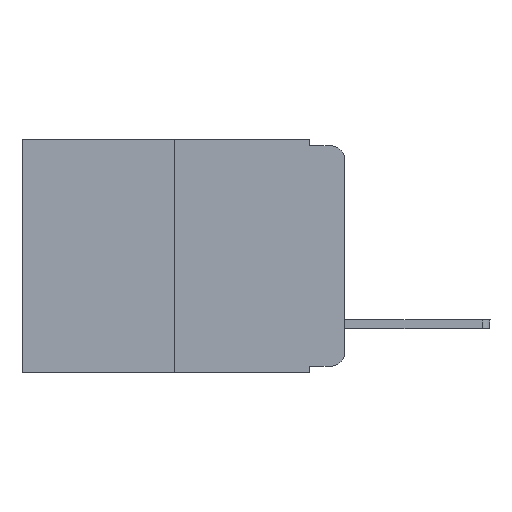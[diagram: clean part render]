
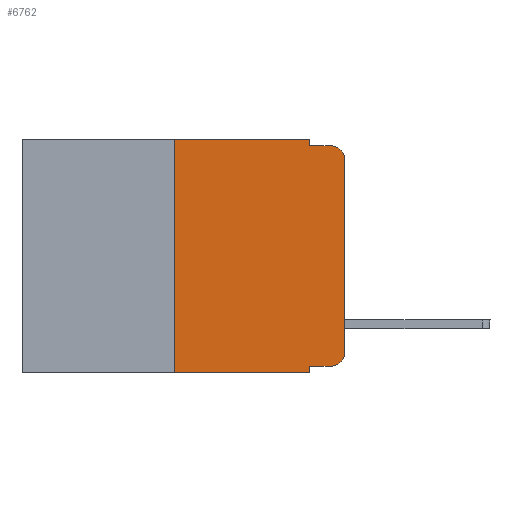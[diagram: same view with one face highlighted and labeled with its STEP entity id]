
A CAD part, left-side view. The second image highlights one B-rep face of the part: STEP entity #6762.
In plain terms, the highlighted planar face has unit normal (-1, 0, 0).
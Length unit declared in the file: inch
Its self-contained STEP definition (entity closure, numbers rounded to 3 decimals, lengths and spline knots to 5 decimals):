
#188 = DIRECTION ( 'NONE',  ( 0., 0., -1. ) ) ;
#242 = VERTEX_POINT ( 'NONE', #1727 ) ;
#404 = CARTESIAN_POINT ( 'NONE',  ( 0., 0.051, -0.333 ) ) ;
#456 = DIRECTION ( 'NONE',  ( 0., -1., 0. ) ) ;
#574 = CARTESIAN_POINT ( 'NONE',  ( 0., 0.051, -0.333 ) ) ;
#636 = CIRCLE ( 'NONE', #5539, 0.02 ) ;
#648 = ORIENTED_EDGE ( 'NONE', *, *, #1151, .T. ) ;
#709 = CARTESIAN_POINT ( 'NONE',  ( 0., 0.473, -0.343 ) ) ;
#1151 = EDGE_CURVE ( 'NONE', #2383, #10334, #2845, .T. ) ;
#1341 = ORIENTED_EDGE ( 'NONE', *, *, #10934, .T. ) ;
#1412 = LINE ( 'NONE', #11946, #2308 ) ;
#1526 = CARTESIAN_POINT ( 'NONE',  ( 0., 0.051, -0.343 ) ) ;
#1555 = EDGE_CURVE ( 'NONE', #3421, #242, #8711, .T. ) ;
#1727 = CARTESIAN_POINT ( 'NONE',  ( 0., 0.02, -0.01 ) ) ;
#1807 = DIRECTION ( 'NONE',  ( 0., 0., 1. ) ) ;
#2109 = PLANE ( 'NONE',  #3914 ) ;
#2184 = LINE ( 'NONE', #3791, #13083 ) ;
#2257 = ORIENTED_EDGE ( 'NONE', *, *, #10537, .T. ) ;
#2308 = VECTOR ( 'NONE', #14338, 39.37008 ) ;
#2383 = VERTEX_POINT ( 'NONE', #5922 ) ;
#2496 = EDGE_CURVE ( 'NONE', #4998, #8439, #12102, .T. ) ;
#2743 = DIRECTION ( 'NONE',  ( 0., 0., -1. ) ) ;
#2845 = LINE ( 'NONE', #709, #11628 ) ;
#2914 = CARTESIAN_POINT ( 'NONE',  ( 0., 0., -0.03 ) ) ;
#3046 = CARTESIAN_POINT ( 'NONE',  ( 0., 0.02, -0.313 ) ) ;
#3060 = ORIENTED_EDGE ( 'NONE', *, *, #4005, .F. ) ;
#3330 = VECTOR ( 'NONE', #5082, 39.37008 ) ;
#3421 = VERTEX_POINT ( 'NONE', #4710 ) ;
#3791 = CARTESIAN_POINT ( 'NONE',  ( 0., 0.25, 0. ) ) ;
#3914 = AXIS2_PLACEMENT_3D ( 'NONE', #9984, #4174, #4481 ) ;
#4005 = EDGE_CURVE ( 'NONE', #4998, #10334, #1412, .T. ) ;
#4174 = DIRECTION ( 'NONE',  ( 1., 0., 0. ) ) ;
#4481 = DIRECTION ( 'NONE',  ( 0., 0., -1. ) ) ;
#4495 = VECTOR ( 'NONE', #14294, 39.37008 ) ;
#4710 = CARTESIAN_POINT ( 'NONE',  ( 0., 0.051, -0.01 ) ) ;
#4913 = CARTESIAN_POINT ( 'NONE',  ( 0., 0., -0.313 ) ) ;
#4998 = VERTEX_POINT ( 'NONE', #574 ) ;
#5045 = VECTOR ( 'NONE', #1807, 39.37008 ) ;
#5082 = DIRECTION ( 'NONE',  ( 0., -1., 0. ) ) ;
#5116 = CARTESIAN_POINT ( 'NONE',  ( 0., 0.473, 0. ) ) ;
#5475 = CARTESIAN_POINT ( 'NONE',  ( 0., 0.02, -0.333 ) ) ;
#5539 = AXIS2_PLACEMENT_3D ( 'NONE', #12075, #8784, #2743 ) ;
#5863 = LINE ( 'NONE', #10586, #12815 ) ;
#5922 = CARTESIAN_POINT ( 'NONE',  ( 0., 0.25, -0.343 ) ) ;
#6175 = CIRCLE ( 'NONE', #8348, 0.02 ) ;
#6287 = EDGE_LOOP ( 'NONE', ( #1341, #2257, #11282, #10245, #12257, #9562, #648, #3060, #12221, #14490 ) ) ;
#6570 = CARTESIAN_POINT ( 'NONE',  ( 0., 0., 0. ) ) ;
#6650 = DIRECTION ( 'NONE',  ( 0., 0., -1. ) ) ;
#6762 = ADVANCED_FACE ( 'NONE', ( #14888 ), #2109, .F. ) ;
#7002 = VECTOR ( 'NONE', #456, 39.37008 ) ;
#7144 = VERTEX_POINT ( 'NONE', #2914 ) ;
#7306 = DIRECTION ( 'NONE',  ( 0., 0., 1. ) ) ;
#7369 = VERTEX_POINT ( 'NONE', #4913 ) ;
#7534 = LINE ( 'NONE', #5116, #4495 ) ;
#7702 = DIRECTION ( 'NONE',  ( -1., 0., 0. ) ) ;
#8348 = AXIS2_PLACEMENT_3D ( 'NONE', #3046, #7702, #6650 ) ;
#8439 = VERTEX_POINT ( 'NONE', #5475 ) ;
#8711 = LINE ( 'NONE', #13386, #7002 ) ;
#8784 = DIRECTION ( 'NONE',  ( -1., 0., 0. ) ) ;
#9562 = ORIENTED_EDGE ( 'NONE', *, *, #13057, .F. ) ;
#9760 = LINE ( 'NONE', #6570, #5045 ) ;
#9984 = CARTESIAN_POINT ( 'NONE',  ( 0., 0.473, 0. ) ) ;
#10059 = EDGE_CURVE ( 'NONE', #12517, #3421, #5863, .T. ) ;
#10245 = ORIENTED_EDGE ( 'NONE', *, *, #10059, .F. ) ;
#10334 = VERTEX_POINT ( 'NONE', #1526 ) ;
#10537 = EDGE_CURVE ( 'NONE', #7144, #242, #636, .T. ) ;
#10586 = CARTESIAN_POINT ( 'NONE',  ( 0., 0.051, 0. ) ) ;
#10837 = CARTESIAN_POINT ( 'NONE',  ( 0., 0.25, 0. ) ) ;
#10934 = EDGE_CURVE ( 'NONE', #7369, #7144, #9760, .T. ) ;
#11105 = DIRECTION ( 'NONE',  ( 0., -1., 0. ) ) ;
#11282 = ORIENTED_EDGE ( 'NONE', *, *, #1555, .F. ) ;
#11439 = EDGE_CURVE ( 'NONE', #11449, #12517, #7534, .T. ) ;
#11449 = VERTEX_POINT ( 'NONE', #10837 ) ;
#11628 = VECTOR ( 'NONE', #11105, 39.37008 ) ;
#11946 = CARTESIAN_POINT ( 'NONE',  ( 0., 0.051, 0. ) ) ;
#12075 = CARTESIAN_POINT ( 'NONE',  ( 0., 0.02, -0.03 ) ) ;
#12102 = LINE ( 'NONE', #404, #3330 ) ;
#12221 = ORIENTED_EDGE ( 'NONE', *, *, #2496, .T. ) ;
#12257 = ORIENTED_EDGE ( 'NONE', *, *, #11439, .F. ) ;
#12517 = VERTEX_POINT ( 'NONE', #13619 ) ;
#12815 = VECTOR ( 'NONE', #188, 39.37008 ) ;
#13057 = EDGE_CURVE ( 'NONE', #2383, #11449, #2184, .T. ) ;
#13083 = VECTOR ( 'NONE', #7306, 39.37008 ) ;
#13386 = CARTESIAN_POINT ( 'NONE',  ( 0., 0.051, -0.01 ) ) ;
#13619 = CARTESIAN_POINT ( 'NONE',  ( 0., 0.051, 0. ) ) ;
#14161 = EDGE_CURVE ( 'NONE', #8439, #7369, #6175, .T. ) ;
#14294 = DIRECTION ( 'NONE',  ( 0., -1., 0. ) ) ;
#14338 = DIRECTION ( 'NONE',  ( 0., 0., -1. ) ) ;
#14490 = ORIENTED_EDGE ( 'NONE', *, *, #14161, .T. ) ;
#14888 = FACE_OUTER_BOUND ( 'NONE', #6287, .T. ) ;
